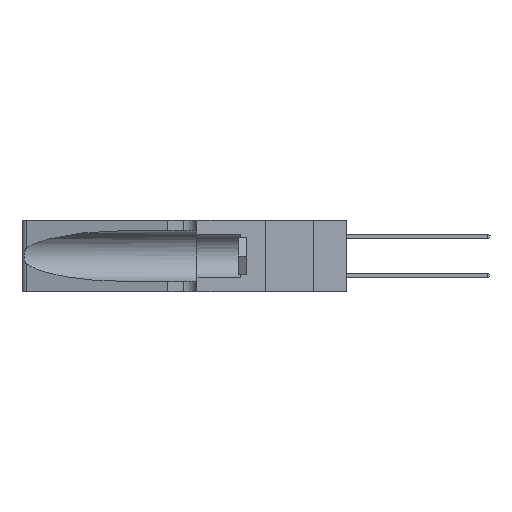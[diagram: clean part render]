
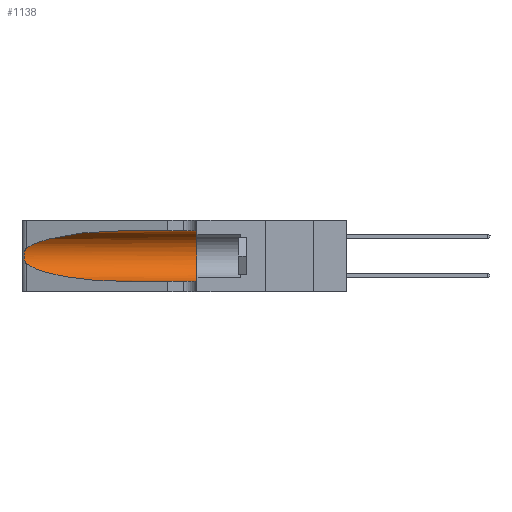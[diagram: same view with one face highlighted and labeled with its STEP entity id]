
A CAD part, left-side view. The second image highlights one B-rep face of the part: STEP entity #1138.
In plain terms, the highlighted cylindrical face has radius 3.308 mm (diameter 6.617 mm), a partial arc.
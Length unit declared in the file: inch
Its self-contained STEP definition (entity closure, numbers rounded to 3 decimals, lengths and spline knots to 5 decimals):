
#5 = LINE ( 'NONE', #16843, #4522 ) ;
#1138 = ADVANCED_FACE ( 'NONE', ( #6955 ), #7537, .F. ) ;
#1139 = CARTESIAN_POINT ( 'NONE',  ( 0.26075, 1.23896, 0.178 ) ) ;
#1228 = VERTEX_POINT ( 'NONE', #11246 ) ;
#2118 = EDGE_CURVE ( 'NONE', #3430, #4910, #7480, .T. ) ;
#2145 = CIRCLE ( 'NONE', #20205, 0.13025 ) ;
#2340 = CARTESIAN_POINT ( 'NONE',  ( 0.25487, 1.22718, 0.14631 ) ) ;
#2357 = EDGE_CURVE ( 'NONE', #21133, #3430, #3060, .T. ) ;
#2638 = VERTEX_POINT ( 'NONE', #9478 ) ;
#2996 = CARTESIAN_POINT ( 'NONE',  ( 0.25555, 1.22994, 0.2215 ) ) ;
#3060 = B_SPLINE_CURVE_WITH_KNOTS ( 'NONE', 3,
 ( #4948, #2996, #8706, #21711, #10558, #23550, #12453, #1139, #14343, #3089, #16211, #5020, #18084, #6924 ),
 .UNSPECIFIED., .F., .F.,
 ( 4, 2, 2, 2, 2, 2, 4 ),
 ( 0., 0.00027, 0.00053, 0.00107, 0.0016, 0.00187, 0.00214 ),
 .UNSPECIFIED. ) ;
#3089 = CARTESIAN_POINT ( 'NONE',  ( 0.25856, 1.23593, 0.16098 ) ) ;
#3369 = VERTEX_POINT ( 'NONE', #9692 ) ;
#3430 = VERTEX_POINT ( 'NONE', #17373 ) ;
#3783 = DIRECTION ( 'NONE',  ( 0., 1., 0. ) ) ;
#4522 = VECTOR ( 'NONE', #7549, 39.37008 ) ;
#4559 = CARTESIAN_POINT ( 'NONE',  ( 0.1305, 0.72297, 0.05475 ) ) ;
#4910 = VERTEX_POINT ( 'NONE', #4559 ) ;
#4948 = CARTESIAN_POINT ( 'NONE',  ( 0.25487, 1.22718, 0.22369 ) ) ;
#5020 = CARTESIAN_POINT ( 'NONE',  ( 0.25639, 1.23186, 0.15144 ) ) ;
#5658 =( BOUNDED_CURVE ( )  B_SPLINE_CURVE ( 3, ( #13205, #9414, #16953, #5758 ),
 .UNSPECIFIED., .F., .T. ) 
 B_SPLINE_CURVE_WITH_KNOTS ( ( 4, 4 ),
 ( 1.5708, 2.84003 ),
 .UNSPECIFIED. ) 
 CURVE ( )  GEOMETRIC_REPRESENTATION_ITEM ( )  RATIONAL_B_SPLINE_CURVE ( ( 1., 0.87, 0.87, 1. ) ) 
 REPRESENTATION_ITEM ( '' )  );
#5758 = CARTESIAN_POINT ( 'NONE',  ( 0.25487, 1.22718, 0.22369 ) ) ;
#6162 = EDGE_CURVE ( 'NONE', #1228, #2638, #2145, .T. ) ;
#6924 = CARTESIAN_POINT ( 'NONE',  ( 0.25487, 1.22718, 0.14631 ) ) ;
#6955 = FACE_OUTER_BOUND ( 'NONE', #16374, .T. ) ;
#7274 = LINE ( 'NONE', #7936, #21521 ) ;
#7480 =( BOUNDED_CURVE ( )  B_SPLINE_CURVE ( 3, ( #2340, #13605, #21008, #15501 ),
 .UNSPECIFIED., .F., .T. ) 
 B_SPLINE_CURVE_WITH_KNOTS ( ( 4, 4 ),
 ( 3.44316, 4.71239 ),
 .UNSPECIFIED. ) 
 CURVE ( )  GEOMETRIC_REPRESENTATION_ITEM ( )  RATIONAL_B_SPLINE_CURVE ( ( 1., 0.87, 0.87, 1. ) ) 
 REPRESENTATION_ITEM ( '' )  );
#7537 = CYLINDRICAL_SURFACE ( 'NONE', #22240, 0.13025 ) ;
#7549 = DIRECTION ( 'NONE',  ( 0., -1., 0. ) ) ;
#7936 = CARTESIAN_POINT ( 'NONE',  ( 0.1305, 1.61858, 0.31525 ) ) ;
#8706 = CARTESIAN_POINT ( 'NONE',  ( 0.25639, 1.23184, 0.21858 ) ) ;
#9060 = ORIENTED_EDGE ( 'NONE', *, *, #13886, .T. ) ;
#9414 = CARTESIAN_POINT ( 'NONE',  ( 0.18966, 0.96281, 0.31525 ) ) ;
#9478 = CARTESIAN_POINT ( 'NONE',  ( 0.1305, 0.35, 0.05475 ) ) ;
#9588 = ORIENTED_EDGE ( 'NONE', *, *, #16108, .T. ) ;
#9692 = CARTESIAN_POINT ( 'NONE',  ( 0.1305, 0.72297, 0.31525 ) ) ;
#10558 = CARTESIAN_POINT ( 'NONE',  ( 0.25854, 1.2359, 0.20912 ) ) ;
#11246 = CARTESIAN_POINT ( 'NONE',  ( 0.1305, 0.35, 0.31525 ) ) ;
#11339 = ORIENTED_EDGE ( 'NONE', *, *, #6162, .F. ) ;
#11614 = CARTESIAN_POINT ( 'NONE',  ( 0.25487, 1.22718, 0.22369 ) ) ;
#12248 = ORIENTED_EDGE ( 'NONE', *, *, #22768, .F. ) ;
#12453 = CARTESIAN_POINT ( 'NONE',  ( 0.26075, 1.23896, 0.19203 ) ) ;
#13205 = CARTESIAN_POINT ( 'NONE',  ( 0.1305, 0.72297, 0.31525 ) ) ;
#13605 = CARTESIAN_POINT ( 'NONE',  ( 0.2373, 1.15595, 0.08982 ) ) ;
#13886 = EDGE_CURVE ( 'NONE', #4910, #2638, #5, .T. ) ;
#14343 = CARTESIAN_POINT ( 'NONE',  ( 0.26017, 1.23833, 0.17102 ) ) ;
#14440 = ORIENTED_EDGE ( 'NONE', *, *, #2357, .T. ) ;
#14991 = CARTESIAN_POINT ( 'NONE',  ( 0.1305, 0.35, 0.185 ) ) ;
#15501 = CARTESIAN_POINT ( 'NONE',  ( 0.1305, 0.72297, 0.05475 ) ) ;
#16108 = EDGE_CURVE ( 'NONE', #3369, #21133, #5658, .T. ) ;
#16211 = CARTESIAN_POINT ( 'NONE',  ( 0.25789, 1.23486, 0.15765 ) ) ;
#16374 = EDGE_LOOP ( 'NONE', ( #9588, #14440, #20934, #9060, #11339, #12248 ) ) ;
#16843 = CARTESIAN_POINT ( 'NONE',  ( 0.1305, 1.61858, 0.05475 ) ) ;
#16875 = DIRECTION ( 'NONE',  ( 0., 0., 1. ) ) ;
#16953 = CARTESIAN_POINT ( 'NONE',  ( 0.2373, 1.15595, 0.28018 ) ) ;
#17229 = DIRECTION ( 'NONE',  ( 0., -1., 0. ) ) ;
#17373 = CARTESIAN_POINT ( 'NONE',  ( 0.25487, 1.22718, 0.14631 ) ) ;
#18084 = CARTESIAN_POINT ( 'NONE',  ( 0.25555, 1.22993, 0.14849 ) ) ;
#18911 = CARTESIAN_POINT ( 'NONE',  ( 0.1305, 1.61858, 0.185 ) ) ;
#19193 = DIRECTION ( 'NONE',  ( 0., -1., 0. ) ) ;
#19324 = DIRECTION ( 'NONE',  ( 0., 0., -1. ) ) ;
#20205 = AXIS2_PLACEMENT_3D ( 'NONE', #14991, #3783, #16875 ) ;
#20934 = ORIENTED_EDGE ( 'NONE', *, *, #2118, .T. ) ;
#21008 = CARTESIAN_POINT ( 'NONE',  ( 0.18966, 0.96281, 0.05475 ) ) ;
#21133 = VERTEX_POINT ( 'NONE', #11614 ) ;
#21521 = VECTOR ( 'NONE', #17229, 39.37008 ) ;
#21711 = CARTESIAN_POINT ( 'NONE',  ( 0.25787, 1.23484, 0.2124 ) ) ;
#22240 = AXIS2_PLACEMENT_3D ( 'NONE', #18911, #19193, #19324 ) ;
#22768 = EDGE_CURVE ( 'NONE', #3369, #1228, #7274, .T. ) ;
#23550 = CARTESIAN_POINT ( 'NONE',  ( 0.26018, 1.23835, 0.19895 ) ) ;
